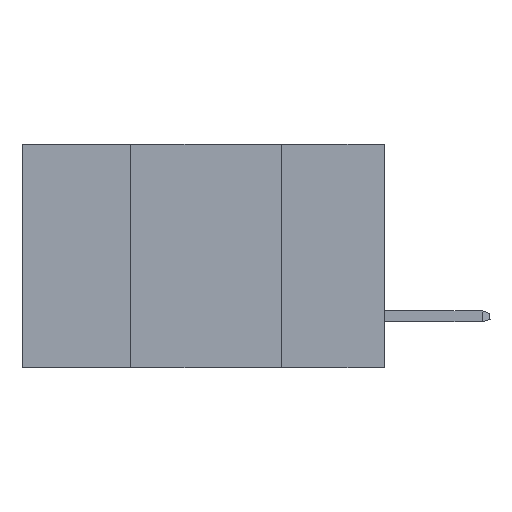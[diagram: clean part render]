
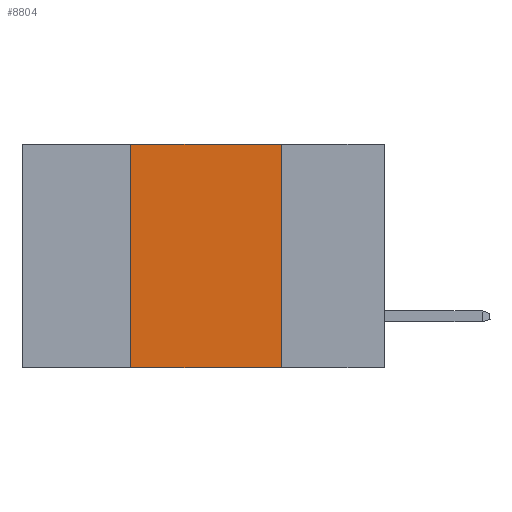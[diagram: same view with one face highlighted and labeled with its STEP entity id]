
A CAD part, left-side view. The second image highlights one B-rep face of the part: STEP entity #8804.
In plain terms, the highlighted planar face has unit normal (-1, 0, 0).
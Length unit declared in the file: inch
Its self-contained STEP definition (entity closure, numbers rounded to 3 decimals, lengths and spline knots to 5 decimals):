
#65 = AXIS2_PLACEMENT_3D ( 'NONE', #10490, #11612, #11738 ) ;
#530 = VERTEX_POINT ( 'NONE', #14138 ) ;
#698 = ORIENTED_EDGE ( 'NONE', *, *, #1431, .F. ) ;
#881 = EDGE_LOOP ( 'NONE', ( #698, #7004, #13340, #6469 ) ) ;
#1117 = CARTESIAN_POINT ( 'NONE',  ( 0., 0.42, 0. ) ) ;
#1173 = LINE ( 'NONE', #5598, #1890 ) ;
#1431 = EDGE_CURVE ( 'NONE', #6725, #530, #14078, .T. ) ;
#1478 = DIRECTION ( 'NONE',  ( 0., -1., 0. ) ) ;
#1490 = CARTESIAN_POINT ( 'NONE',  ( 0., 0.17, 0. ) ) ;
#1730 = CARTESIAN_POINT ( 'NONE',  ( 0., 0.17, 0. ) ) ;
#1890 = VECTOR ( 'NONE', #8867, 39.37008 ) ;
#1908 = PLANE ( 'NONE',  #65 ) ;
#4392 = DIRECTION ( 'NONE',  ( 0., 0., 1. ) ) ;
#4447 = LINE ( 'NONE', #1117, #12138 ) ;
#5257 = EDGE_CURVE ( 'NONE', #11260, #6725, #13192, .T. ) ;
#5598 = CARTESIAN_POINT ( 'NONE',  ( 0., 0.6, -0.37 ) ) ;
#5812 = CARTESIAN_POINT ( 'NONE',  ( 0., 0.6, 0. ) ) ;
#6469 = ORIENTED_EDGE ( 'NONE', *, *, #13027, .T. ) ;
#6725 = VERTEX_POINT ( 'NONE', #1490 ) ;
#7004 = ORIENTED_EDGE ( 'NONE', *, *, #5257, .F. ) ;
#7592 = VECTOR ( 'NONE', #10639, 39.37008 ) ;
#8064 = VECTOR ( 'NONE', #1478, 39.37008 ) ;
#8804 = ADVANCED_FACE ( 'NONE', ( #10526 ), #1908, .F. ) ;
#8867 = DIRECTION ( 'NONE',  ( 0., -1., 0. ) ) ;
#9220 = VERTEX_POINT ( 'NONE', #12383 ) ;
#10490 = CARTESIAN_POINT ( 'NONE',  ( 0., 0.6, 0. ) ) ;
#10526 = FACE_OUTER_BOUND ( 'NONE', #881, .T. ) ;
#10639 = DIRECTION ( 'NONE',  ( 0., 0., -1. ) ) ;
#11260 = VERTEX_POINT ( 'NONE', #11508 ) ;
#11508 = CARTESIAN_POINT ( 'NONE',  ( 0., 0.42, 0. ) ) ;
#11612 = DIRECTION ( 'NONE',  ( 1., 0., 0. ) ) ;
#11738 = DIRECTION ( 'NONE',  ( 0., 0., -1. ) ) ;
#12138 = VECTOR ( 'NONE', #4392, 39.37008 ) ;
#12383 = CARTESIAN_POINT ( 'NONE',  ( 0., 0.42, -0.37 ) ) ;
#13027 = EDGE_CURVE ( 'NONE', #9220, #530, #1173, .T. ) ;
#13184 = EDGE_CURVE ( 'NONE', #9220, #11260, #4447, .T. ) ;
#13192 = LINE ( 'NONE', #5812, #8064 ) ;
#13340 = ORIENTED_EDGE ( 'NONE', *, *, #13184, .F. ) ;
#14078 = LINE ( 'NONE', #1730, #7592 ) ;
#14138 = CARTESIAN_POINT ( 'NONE',  ( 0., 0.17, -0.37 ) ) ;
